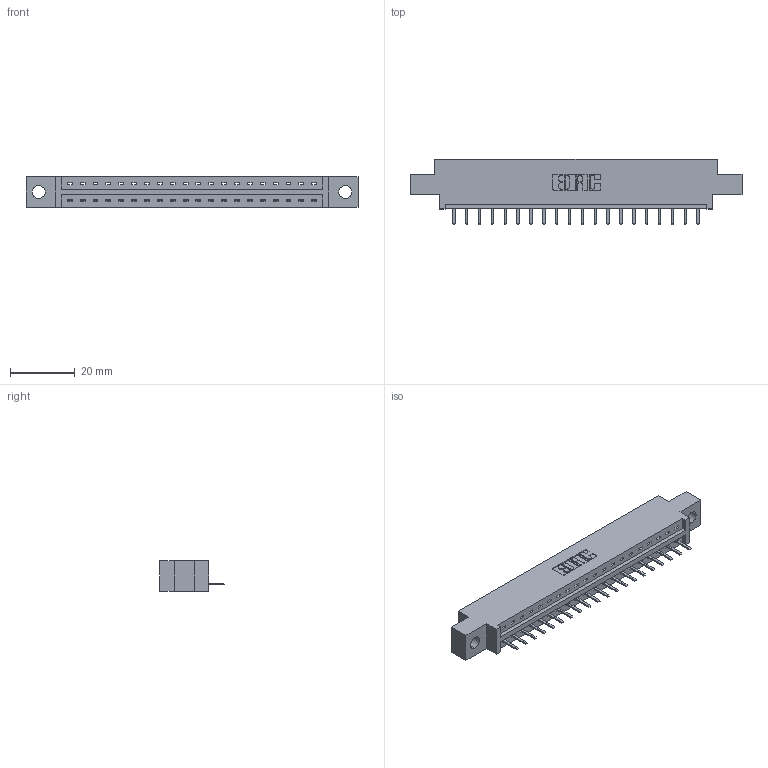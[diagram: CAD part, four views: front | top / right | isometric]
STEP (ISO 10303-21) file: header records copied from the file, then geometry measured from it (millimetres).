
FILE_DESCRIPTION (( 'STEP AP203' ), '1' );
FILE_NAME ('387-020-520-604.STEP', '2019-10-02T22:06:12', ( '' ), ( '' ), 'SwSTEP 2.0', 'SolidWorks 2016', '' );
FILE_SCHEMA (( 'CONFIG_CONTROL_DESIGN' ));
Length unit declared in the file: inch
Products named in the file (3): 337 Part_0.170 Offset - 0.156 Dia-TH; 345-292-001_345-293-120; 387-020-520-604
Assembly tree (21 placements, depth 2):
  387-020-520-604
    337 Part_0.170 Offset - 0.156 Dia-TH
    345-292-001_345-293-120  x20
Bounding box: 102.26 x 20.02 x 9.4 mm (x, y, z)
Volume: 10090.1 mm3; surface area: 9989.1 mm2
Topology: 21 solids, 21 shells, 1438 faces, 4243 edges, 2774 vertices
Faces by surface type: plane 1034, cylinder 404
Entity records: 17961 total; most frequent: CARTESIAN_POINT 3146, ORIENTED_EDGE 3090, DIRECTION 2681, EDGE_CURVE 1545, VECTOR 1413, LINE 1413, VERTEX_POINT 1026, AXIS2_PLACEMENT_3D 634
